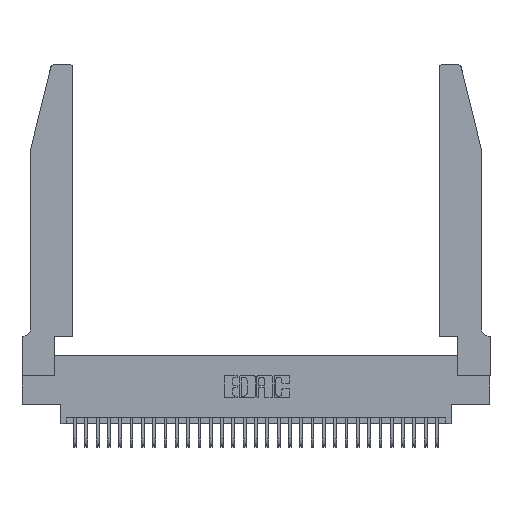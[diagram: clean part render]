
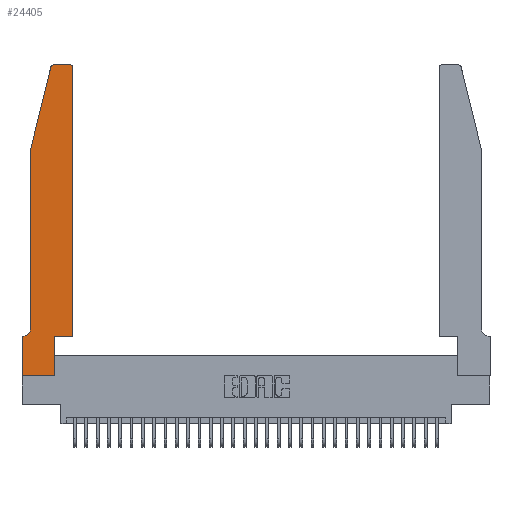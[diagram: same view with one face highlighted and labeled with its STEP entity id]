
A CAD part, top view. The second image highlights one B-rep face of the part: STEP entity #24405.
In plain terms, the highlighted planar face has unit normal (0, 0, 1).
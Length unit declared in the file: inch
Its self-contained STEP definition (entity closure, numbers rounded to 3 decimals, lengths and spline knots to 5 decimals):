
#86 = DIRECTION ( 'NONE',  ( 1., 0., 0. ) ) ;
#188 = CARTESIAN_POINT ( 'NONE',  ( 0.0755, 0.35, 0.37 ) ) ;
#618 = EDGE_CURVE ( 'NONE', #4739, #26035, #3175, .T. ) ;
#641 = ORIENTED_EDGE ( 'NONE', *, *, #1108, .T. ) ;
#937 = DIRECTION ( 'NONE',  ( 0., 0., 1. ) ) ;
#1108 = EDGE_CURVE ( 'NONE', #29070, #4739, #33216, .T. ) ;
#1162 = CARTESIAN_POINT ( 'NONE',  ( 0.0055, 0.35, 0.37 ) ) ;
#1534 = EDGE_CURVE ( 'NONE', #25838, #16108, #24562, .T. ) ;
#2056 = CARTESIAN_POINT ( 'NONE',  ( 0.4505, 0.35, 0.37 ) ) ;
#2327 = EDGE_CURVE ( 'NONE', #16108, #11047, #31612, .T. ) ;
#2951 = LINE ( 'NONE', #16969, #23061 ) ;
#3175 = LINE ( 'NONE', #11029, #29982 ) ;
#3210 = VERTEX_POINT ( 'NONE', #31385 ) ;
#3540 = CARTESIAN_POINT ( 'NONE',  ( 0.0755, 2., 0.37 ) ) ;
#3554 = CARTESIAN_POINT ( 'NONE',  ( 0.0755, 0.42, 0.37 ) ) ;
#3916 = ORIENTED_EDGE ( 'NONE', *, *, #27295, .T. ) ;
#3991 = ORIENTED_EDGE ( 'NONE', *, *, #29104, .T. ) ;
#4163 = CARTESIAN_POINT ( 'NONE',  ( 0., 0., 0.37 ) ) ;
#4306 = VECTOR ( 'NONE', #14860, 39.37008 ) ;
#4392 = DIRECTION ( 'NONE',  ( 0., 0., -1. ) ) ;
#4640 = ORIENTED_EDGE ( 'NONE', *, *, #8223, .T. ) ;
#4739 = VERTEX_POINT ( 'NONE', #2056 ) ;
#5424 = AXIS2_PLACEMENT_3D ( 'NONE', #31318, #16066, #86 ) ;
#6672 = CARTESIAN_POINT ( 'NONE',  ( 0.2865, 0.35, 0.37 ) ) ;
#6903 = DIRECTION ( 'NONE',  ( 1., 0., 0. ) ) ;
#7547 = CARTESIAN_POINT ( 'NONE',  ( 0.4505, 0.35, 0.37 ) ) ;
#8007 = CARTESIAN_POINT ( 'NONE',  ( 0.0755, 2., 0.37 ) ) ;
#8205 = EDGE_CURVE ( 'NONE', #11047, #3210, #2951, .T. ) ;
#8223 = EDGE_CURVE ( 'NONE', #23176, #25838, #16213, .T. ) ;
#9553 = DIRECTION ( 'NONE',  ( 0., 1., 0. ) ) ;
#10049 = EDGE_CURVE ( 'NONE', #20082, #22930, #32791, .T. ) ;
#10552 = DIRECTION ( 'NONE',  ( 0., 0., 1. ) ) ;
#10569 = CARTESIAN_POINT ( 'NONE',  ( 0.284, 2.75, 0.37 ) ) ;
#11029 = CARTESIAN_POINT ( 'NONE',  ( 0.4505, 0.35, 0.37 ) ) ;
#11047 = VERTEX_POINT ( 'NONE', #25882 ) ;
#11214 = AXIS2_PLACEMENT_3D ( 'NONE', #26024, #10552, #28566 ) ;
#11701 = DIRECTION ( 'NONE',  ( 1., 0., 0. ) ) ;
#11827 = CARTESIAN_POINT ( 'NONE',  ( 0.2605, 2.75, 0.37 ) ) ;
#12294 = VECTOR ( 'NONE', #23619, 39.37008 ) ;
#12404 = ORIENTED_EDGE ( 'NONE', *, *, #12414, .T. ) ;
#12414 = EDGE_CURVE ( 'NONE', #26035, #20082, #26730, .T. ) ;
#12681 = VERTEX_POINT ( 'NONE', #3540 ) ;
#13502 = ORIENTED_EDGE ( 'NONE', *, *, #24785, .T. ) ;
#14089 = VECTOR ( 'NONE', #30275, 39.37008 ) ;
#14198 = DIRECTION ( 'NONE',  ( -1., 0., 0. ) ) ;
#14860 = DIRECTION ( 'NONE',  ( 0., 1., 0. ) ) ;
#15911 = CIRCLE ( 'NONE', #5424, 0.03 ) ;
#16066 = DIRECTION ( 'NONE',  ( 0., 0., 1. ) ) ;
#16108 = VERTEX_POINT ( 'NONE', #22591 ) ;
#16213 = CIRCLE ( 'NONE', #33224, 0.07 ) ;
#16831 = FACE_OUTER_BOUND ( 'NONE', #17424, .T. ) ;
#16888 = CARTESIAN_POINT ( 'NONE',  ( 0., 0.35, 0.37 ) ) ;
#16940 = EDGE_CURVE ( 'NONE', #3210, #29070, #25134, .T. ) ;
#16942 = VECTOR ( 'NONE', #14198, 39.37008 ) ;
#16969 = CARTESIAN_POINT ( 'NONE',  ( 0., 0., 0.37 ) ) ;
#17340 = ORIENTED_EDGE ( 'NONE', *, *, #10049, .T. ) ;
#17424 = EDGE_LOOP ( 'NONE', ( #17340, #3916, #13502, #3991, #4640, #22554, #22500, #23343, #28852, #641, #17711, #12404 ) ) ;
#17711 = ORIENTED_EDGE ( 'NONE', *, *, #618, .T. ) ;
#18137 = VECTOR ( 'NONE', #32530, 39.37008 ) ;
#18382 = AXIS2_PLACEMENT_3D ( 'NONE', #16888, #937, #19479 ) ;
#19479 = DIRECTION ( 'NONE',  ( 1., 0., 0. ) ) ;
#20064 = CARTESIAN_POINT ( 'NONE',  ( 0.0755, 2., 0.37 ) ) ;
#20082 = VERTEX_POINT ( 'NONE', #28055 ) ;
#20122 = CARTESIAN_POINT ( 'NONE',  ( 0.0055, 0.42, 0.37 ) ) ;
#21021 = LINE ( 'NONE', #20064, #14089 ) ;
#22500 = ORIENTED_EDGE ( 'NONE', *, *, #2327, .T. ) ;
#22554 = ORIENTED_EDGE ( 'NONE', *, *, #1534, .T. ) ;
#22591 = CARTESIAN_POINT ( 'NONE',  ( 0., 0.35, 0.37 ) ) ;
#22714 = DIRECTION ( 'NONE',  ( -1., 0., 0. ) ) ;
#22930 = VERTEX_POINT ( 'NONE', #10569 ) ;
#23061 = VECTOR ( 'NONE', #11701, 39.37008 ) ;
#23176 = VERTEX_POINT ( 'NONE', #3554 ) ;
#23343 = ORIENTED_EDGE ( 'NONE', *, *, #8205, .T. ) ;
#23619 = DIRECTION ( 'NONE',  ( -0.239, -0.971, 0. ) ) ;
#24405 = ADVANCED_FACE ( 'NONE', ( #16831 ), #32094, .T. ) ;
#24562 = LINE ( 'NONE', #188, #16942 ) ;
#24704 = DIRECTION ( 'NONE',  ( -1., 0., 0. ) ) ;
#24785 = EDGE_CURVE ( 'NONE', #27514, #12681, #26017, .T. ) ;
#25134 = LINE ( 'NONE', #27637, #4306 ) ;
#25838 = VERTEX_POINT ( 'NONE', #1162 ) ;
#25882 = CARTESIAN_POINT ( 'NONE',  ( 0., 0., 0.37 ) ) ;
#26017 = LINE ( 'NONE', #8007, #12294 ) ;
#26024 = CARTESIAN_POINT ( 'NONE',  ( 0.4205, 2.72, 0.37 ) ) ;
#26035 = VERTEX_POINT ( 'NONE', #33043 ) ;
#26517 = VECTOR ( 'NONE', #6903, 39.37008 ) ;
#26730 = CIRCLE ( 'NONE', #11214, 0.03 ) ;
#26882 = VECTOR ( 'NONE', #24704, 39.37008 ) ;
#26992 = CARTESIAN_POINT ( 'NONE',  ( 0.25487, 2.72718, 0.37 ) ) ;
#27295 = EDGE_CURVE ( 'NONE', #22930, #27514, #15911, .T. ) ;
#27514 = VERTEX_POINT ( 'NONE', #26992 ) ;
#27637 = CARTESIAN_POINT ( 'NONE',  ( 0.2865, 0.35, 0.37 ) ) ;
#28055 = CARTESIAN_POINT ( 'NONE',  ( 0.4205, 2.75, 0.37 ) ) ;
#28566 = DIRECTION ( 'NONE',  ( 1., 0., 0. ) ) ;
#28852 = ORIENTED_EDGE ( 'NONE', *, *, #16940, .T. ) ;
#29070 = VERTEX_POINT ( 'NONE', #6672 ) ;
#29104 = EDGE_CURVE ( 'NONE', #12681, #23176, #21021, .T. ) ;
#29982 = VECTOR ( 'NONE', #9553, 39.37008 ) ;
#30275 = DIRECTION ( 'NONE',  ( 0., -1., 0. ) ) ;
#31318 = CARTESIAN_POINT ( 'NONE',  ( 0.284, 2.72, 0.37 ) ) ;
#31385 = CARTESIAN_POINT ( 'NONE',  ( 0.2865, 0., 0.37 ) ) ;
#31612 = LINE ( 'NONE', #4163, #18137 ) ;
#32094 = PLANE ( 'NONE',  #18382 ) ;
#32530 = DIRECTION ( 'NONE',  ( 0., -1., 0. ) ) ;
#32791 = LINE ( 'NONE', #11827, #26882 ) ;
#33043 = CARTESIAN_POINT ( 'NONE',  ( 0.4505, 2.72, 0.37 ) ) ;
#33216 = LINE ( 'NONE', #7547, #26517 ) ;
#33224 = AXIS2_PLACEMENT_3D ( 'NONE', #20122, #4392, #22714 ) ;
